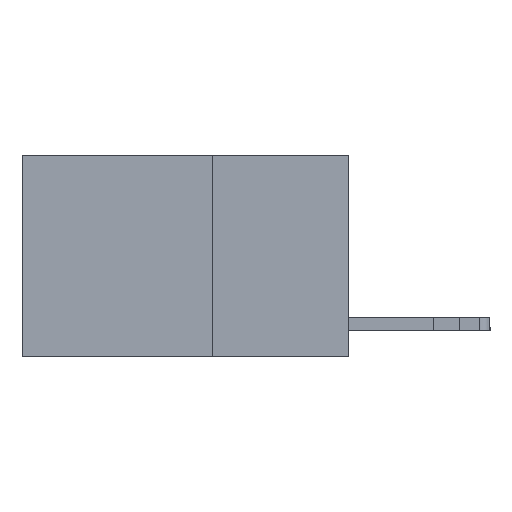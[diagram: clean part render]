
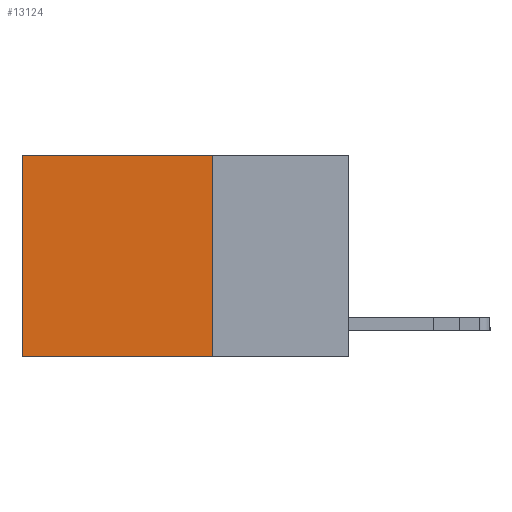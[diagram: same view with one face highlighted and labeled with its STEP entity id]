
A CAD part, left-side view. The second image highlights one B-rep face of the part: STEP entity #13124.
In plain terms, the highlighted planar face has unit normal (-1, 0, 0).
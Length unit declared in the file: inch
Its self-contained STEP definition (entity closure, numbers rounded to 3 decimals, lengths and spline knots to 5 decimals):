
#407 = LINE ( 'NONE', #17966, #5782 ) ;
#1047 = EDGE_CURVE ( 'NONE', #16317, #10859, #6436, .T. ) ;
#1214 = VERTEX_POINT ( 'NONE', #5078 ) ;
#1359 = CARTESIAN_POINT ( 'NONE',  ( 0.2625, 0.6, 0. ) ) ;
#1719 = CARTESIAN_POINT ( 'NONE',  ( 0.2625, 0.6, -0.37 ) ) ;
#2405 = CARTESIAN_POINT ( 'NONE',  ( 0.2625, 0.25, 0. ) ) ;
#3992 = EDGE_LOOP ( 'NONE', ( #16679, #6623, #20037, #5283 ) ) ;
#5078 = CARTESIAN_POINT ( 'NONE',  ( 0.2625, 0.25, -0.37 ) ) ;
#5283 = ORIENTED_EDGE ( 'NONE', *, *, #1047, .T. ) ;
#5394 = EDGE_CURVE ( 'NONE', #10859, #7646, #407, .T. ) ;
#5448 = AXIS2_PLACEMENT_3D ( 'NONE', #2405, #14738, #17961 ) ;
#5782 = VECTOR ( 'NONE', #11915, 39.37008 ) ;
#5888 = DIRECTION ( 'NONE',  ( 0., 1., 0. ) ) ;
#6436 = LINE ( 'NONE', #17268, #10961 ) ;
#6623 = ORIENTED_EDGE ( 'NONE', *, *, #7902, .F. ) ;
#7529 = LINE ( 'NONE', #20265, #15631 ) ;
#7646 = VERTEX_POINT ( 'NONE', #1719 ) ;
#7902 = EDGE_CURVE ( 'NONE', #1214, #7646, #13743, .T. ) ;
#10184 = VECTOR ( 'NONE', #5888, 39.37008 ) ;
#10557 = DIRECTION ( 'NONE',  ( 0., 0., -1. ) ) ;
#10859 = VERTEX_POINT ( 'NONE', #1359 ) ;
#10961 = VECTOR ( 'NONE', #17367, 39.37008 ) ;
#11915 = DIRECTION ( 'NONE',  ( 0., 0., -1. ) ) ;
#13124 = ADVANCED_FACE ( 'NONE', ( #13497 ), #19854, .F. ) ;
#13497 = FACE_OUTER_BOUND ( 'NONE', #3992, .T. ) ;
#13743 = LINE ( 'NONE', #18332, #10184 ) ;
#14738 = DIRECTION ( 'NONE',  ( 1., 0., 0. ) ) ;
#15631 = VECTOR ( 'NONE', #10557, 39.37008 ) ;
#16317 = VERTEX_POINT ( 'NONE', #20655 ) ;
#16679 = ORIENTED_EDGE ( 'NONE', *, *, #5394, .T. ) ;
#17179 = EDGE_CURVE ( 'NONE', #16317, #1214, #7529, .T. ) ;
#17268 = CARTESIAN_POINT ( 'NONE',  ( 0.2625, 0.25, 0. ) ) ;
#17367 = DIRECTION ( 'NONE',  ( 0., 1., 0. ) ) ;
#17961 = DIRECTION ( 'NONE',  ( 0., 0., -1. ) ) ;
#17966 = CARTESIAN_POINT ( 'NONE',  ( 0.2625, 0.6, 0. ) ) ;
#18332 = CARTESIAN_POINT ( 'NONE',  ( 0.2625, 0.25, -0.37 ) ) ;
#19854 = PLANE ( 'NONE',  #5448 ) ;
#20037 = ORIENTED_EDGE ( 'NONE', *, *, #17179, .F. ) ;
#20265 = CARTESIAN_POINT ( 'NONE',  ( 0.2625, 0.25, 0. ) ) ;
#20655 = CARTESIAN_POINT ( 'NONE',  ( 0.2625, 0.25, 0. ) ) ;
